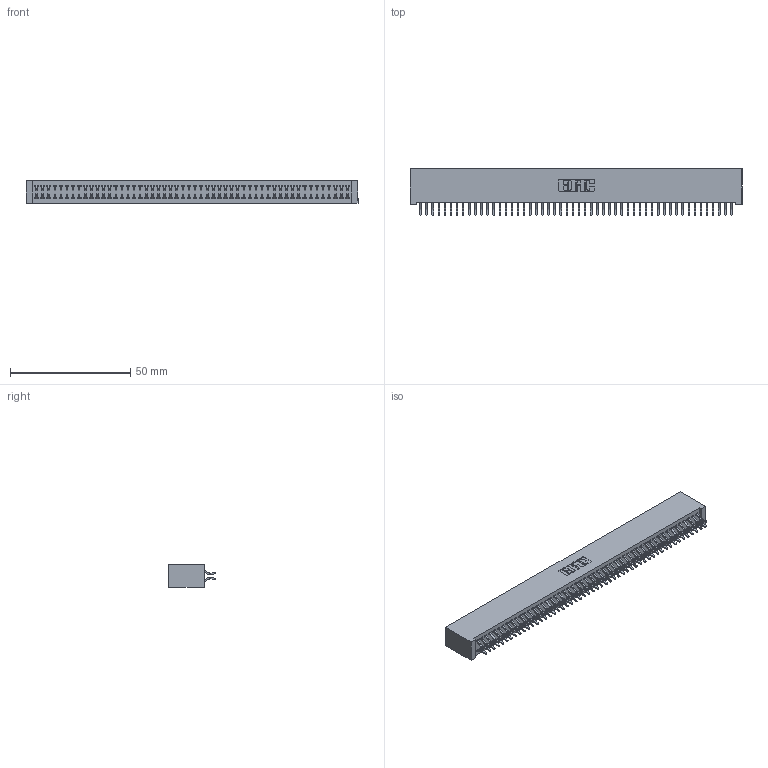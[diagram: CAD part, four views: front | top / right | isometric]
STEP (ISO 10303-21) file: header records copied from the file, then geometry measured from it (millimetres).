
FILE_DESCRIPTION (( 'STEP AP203' ), '1' );
FILE_NAME ('342-104-556-201.STEP', '2019-10-04T18:50:37', ( '' ), ( '' ), 'SwSTEP 2.0', 'SolidWorks 2016', '' );
FILE_SCHEMA (( 'CONFIG_CONTROL_DESIGN' ));
Length unit declared in the file: inch
Products named in the file (3): 342 Part_Lugless; 342-104-556-201; 345-292-001_556 Tail
Assembly tree (105 placements, depth 2):
  342-104-556-201
    342 Part_Lugless
    345-292-001_556 Tail  x104
Bounding box: 138.33 x 19.58 x 9.4 mm (x, y, z)
Volume: 12913 mm3; surface area: 21610.9 mm2
Topology: 105 solids, 105 shells, 6134 faces, 18267 edges, 12038 vertices
Faces by surface type: plane 4222, cylinder 1912
Entity records: 31971 total; most frequent: CARTESIAN_POINT 5298, ORIENTED_EDGE 5222, DIRECTION 4491, EDGE_CURVE 2611, VECTOR 2483, LINE 2483, VERTEX_POINT 1738, AXIS2_PLACEMENT_3D 1004
